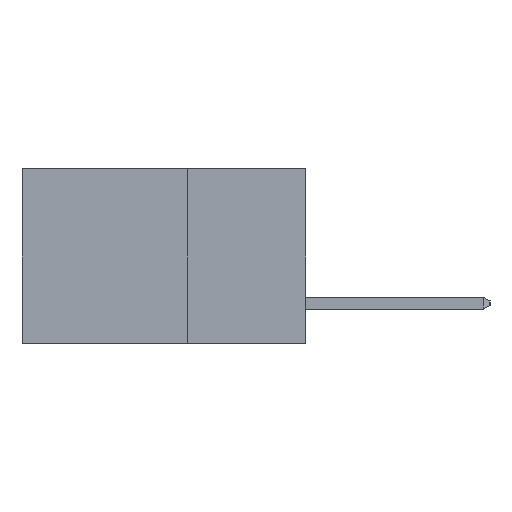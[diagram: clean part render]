
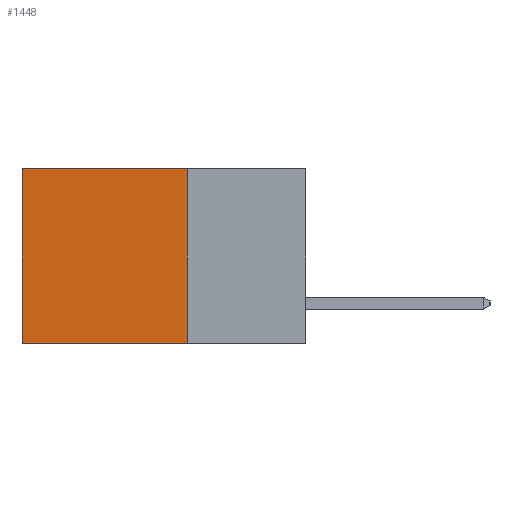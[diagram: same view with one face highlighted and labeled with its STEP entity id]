
A CAD part, left-side view. The second image highlights one B-rep face of the part: STEP entity #1448.
In plain terms, the highlighted planar face has unit normal (-1, 0, 0).
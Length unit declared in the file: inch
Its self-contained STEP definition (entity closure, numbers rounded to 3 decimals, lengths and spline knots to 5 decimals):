
#199 = CARTESIAN_POINT ( 'NONE',  ( 0.2615, 0.25, 0. ) ) ;
#202 = ORIENTED_EDGE ( 'NONE', *, *, #2920, .T. ) ;
#772 = EDGE_CURVE ( 'NONE', #16140, #12234, #13570, .T. ) ;
#1357 = LINE ( 'NONE', #3001, #8165 ) ;
#1448 = ADVANCED_FACE ( 'NONE', ( #8728 ), #9538, .F. ) ;
#1859 = ORIENTED_EDGE ( 'NONE', *, *, #772, .T. ) ;
#1897 = CARTESIAN_POINT ( 'NONE',  ( 0.2615, 0.25, -0.37 ) ) ;
#2920 = EDGE_CURVE ( 'NONE', #12234, #4266, #1357, .T. ) ;
#3001 = CARTESIAN_POINT ( 'NONE',  ( 0.2615, 0.6, -0.37 ) ) ;
#3194 = CARTESIAN_POINT ( 'NONE',  ( 0.2615, 0.6, -0.37 ) ) ;
#3214 = DIRECTION ( 'NONE',  ( 1., 0., 0. ) ) ;
#3429 = CARTESIAN_POINT ( 'NONE',  ( 0.2615, 0.25, -0.37 ) ) ;
#4266 = VERTEX_POINT ( 'NONE', #3194 ) ;
#4895 = CARTESIAN_POINT ( 'NONE',  ( 0.2615, 0.25, -0.37 ) ) ;
#5420 = LINE ( 'NONE', #3429, #14808 ) ;
#6142 = DIRECTION ( 'NONE',  ( 0., 0., -1. ) ) ;
#6895 = AXIS2_PLACEMENT_3D ( 'NONE', #1897, #3214, #10337 ) ;
#7725 = DIRECTION ( 'NONE',  ( 0., 1., 0. ) ) ;
#7779 = LINE ( 'NONE', #16541, #11632 ) ;
#8165 = VECTOR ( 'NONE', #10933, 39.37008 ) ;
#8728 = FACE_OUTER_BOUND ( 'NONE', #15061, .T. ) ;
#8736 = EDGE_CURVE ( 'NONE', #16140, #14316, #5420, .T. ) ;
#9538 = PLANE ( 'NONE',  #6895 ) ;
#10337 = DIRECTION ( 'NONE',  ( 0., 0., -1. ) ) ;
#10933 = DIRECTION ( 'NONE',  ( 0., 0., -1. ) ) ;
#11057 = EDGE_CURVE ( 'NONE', #14316, #4266, #7779, .T. ) ;
#11551 = DIRECTION ( 'NONE',  ( 0., 1., 0. ) ) ;
#11632 = VECTOR ( 'NONE', #7725, 39.37008 ) ;
#12101 = ORIENTED_EDGE ( 'NONE', *, *, #11057, .F. ) ;
#12234 = VERTEX_POINT ( 'NONE', #15659 ) ;
#12491 = CARTESIAN_POINT ( 'NONE',  ( 0.2615, 0.25, 0. ) ) ;
#13188 = VECTOR ( 'NONE', #11551, 39.37008 ) ;
#13570 = LINE ( 'NONE', #12491, #13188 ) ;
#14316 = VERTEX_POINT ( 'NONE', #4895 ) ;
#14466 = ORIENTED_EDGE ( 'NONE', *, *, #8736, .F. ) ;
#14808 = VECTOR ( 'NONE', #6142, 39.37008 ) ;
#15061 = EDGE_LOOP ( 'NONE', ( #202, #12101, #14466, #1859 ) ) ;
#15659 = CARTESIAN_POINT ( 'NONE',  ( 0.2615, 0.6, 0. ) ) ;
#16140 = VERTEX_POINT ( 'NONE', #199 ) ;
#16541 = CARTESIAN_POINT ( 'NONE',  ( 0.2615, 0.25, -0.37 ) ) ;
